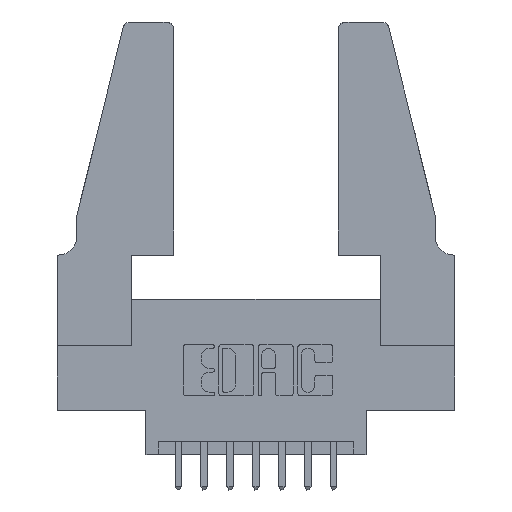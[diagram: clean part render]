
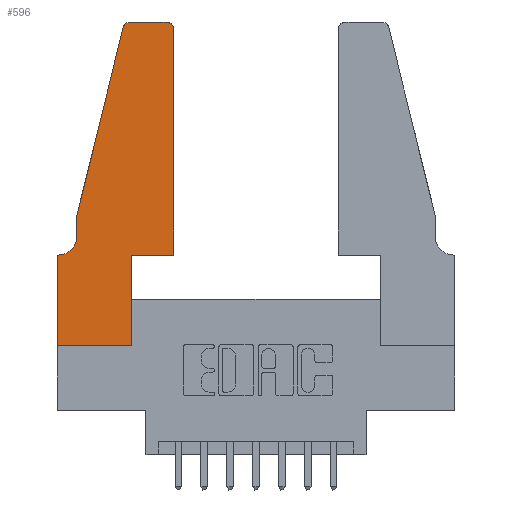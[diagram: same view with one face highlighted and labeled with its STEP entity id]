
A CAD part, top view. The second image highlights one B-rep face of the part: STEP entity #596.
In plain terms, the highlighted planar face has unit normal (0, 0, 1).
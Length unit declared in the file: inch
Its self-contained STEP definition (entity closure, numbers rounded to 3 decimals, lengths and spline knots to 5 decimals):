
#3 = LINE ( 'NONE', #2616, #12503 ) ;
#72 = VECTOR ( 'NONE', #836, 39.37008 ) ;
#285 = VERTEX_POINT ( 'NONE', #7904 ) ;
#545 = CARTESIAN_POINT ( 'NONE',  ( 0., 0., 0.37 ) ) ;
#596 = ADVANCED_FACE ( 'NONE', ( #7240 ), #2497, .T. ) ;
#632 = CIRCLE ( 'NONE', #2357, 0.07 ) ;
#703 = DIRECTION ( 'NONE',  ( 0., -1., 0. ) ) ;
#830 = DIRECTION ( 'NONE',  ( -1., 0., 0. ) ) ;
#836 = DIRECTION ( 'NONE',  ( 1., 0., 0. ) ) ;
#1062 = CARTESIAN_POINT ( 'NONE',  ( 0.0755, 0.42, 0.37 ) ) ;
#1194 = ORIENTED_EDGE ( 'NONE', *, *, #9621, .T. ) ;
#1334 = CARTESIAN_POINT ( 'NONE',  ( 0.4505, 0.35, 0.37 ) ) ;
#1351 = DIRECTION ( 'NONE',  ( 0., 1., 0. ) ) ;
#1478 = CARTESIAN_POINT ( 'NONE',  ( 0.4505, 0.35, 0.37 ) ) ;
#1559 = CARTESIAN_POINT ( 'NONE',  ( 0.4505, 1.22, 0.37 ) ) ;
#1688 = ORIENTED_EDGE ( 'NONE', *, *, #3262, .T. ) ;
#1807 = EDGE_CURVE ( 'NONE', #3341, #2200, #9001, .T. ) ;
#1856 = ORIENTED_EDGE ( 'NONE', *, *, #2678, .T. ) ;
#2013 = EDGE_CURVE ( 'NONE', #2795, #11368, #11263, .T. ) ;
#2200 = VERTEX_POINT ( 'NONE', #1062 ) ;
#2223 = VERTEX_POINT ( 'NONE', #3822 ) ;
#2312 = EDGE_CURVE ( 'NONE', #5438, #7473, #8326, .T. ) ;
#2357 = AXIS2_PLACEMENT_3D ( 'NONE', #5072, #4078, #9927 ) ;
#2497 = PLANE ( 'NONE',  #7299 ) ;
#2530 = CARTESIAN_POINT ( 'NONE',  ( 0.284, 1.22, 0.37 ) ) ;
#2616 = CARTESIAN_POINT ( 'NONE',  ( 0., 0., 0.37 ) ) ;
#2678 = EDGE_CURVE ( 'NONE', #2200, #5438, #632, .T. ) ;
#2680 = VECTOR ( 'NONE', #4739, 39.37008 ) ;
#2780 = ORIENTED_EDGE ( 'NONE', *, *, #2312, .T. ) ;
#2795 = VERTEX_POINT ( 'NONE', #545 ) ;
#3213 = EDGE_CURVE ( 'NONE', #6427, #285, #8364, .T. ) ;
#3262 = EDGE_CURVE ( 'NONE', #12402, #2223, #9408, .T. ) ;
#3292 = ORIENTED_EDGE ( 'NONE', *, *, #2013, .T. ) ;
#3341 = VERTEX_POINT ( 'NONE', #4653 ) ;
#3409 = CARTESIAN_POINT ( 'NONE',  ( 0.2865, 0., 0.37 ) ) ;
#3668 = EDGE_CURVE ( 'NONE', #7473, #2795, #3, .T. ) ;
#3670 = CARTESIAN_POINT ( 'NONE',  ( 0.284, 1.25, 0.37 ) ) ;
#3787 = EDGE_CURVE ( 'NONE', #5782, #5956, #7273, .T. ) ;
#3812 = LINE ( 'NONE', #5232, #6368 ) ;
#3822 = CARTESIAN_POINT ( 'NONE',  ( 0.25487, 1.22718, 0.37 ) ) ;
#3830 = VECTOR ( 'NONE', #9190, 39.37008 ) ;
#3849 = ORIENTED_EDGE ( 'NONE', *, *, #3213, .T. ) ;
#4078 = DIRECTION ( 'NONE',  ( 0., 0., -1. ) ) ;
#4103 = ORIENTED_EDGE ( 'NONE', *, *, #3787, .T. ) ;
#4184 = AXIS2_PLACEMENT_3D ( 'NONE', #5193, #6030, #5018 ) ;
#4193 = DIRECTION ( 'NONE',  ( -0.239, -0.971, 0. ) ) ;
#4235 = ORIENTED_EDGE ( 'NONE', *, *, #3668, .T. ) ;
#4653 = CARTESIAN_POINT ( 'NONE',  ( 0.0755, 0.5, 0.37 ) ) ;
#4739 = DIRECTION ( 'NONE',  ( 0., -1., 0. ) ) ;
#4747 = DIRECTION ( 'NONE',  ( 1., 0., 0. ) ) ;
#5018 = DIRECTION ( 'NONE',  ( 1., 0., 0. ) ) ;
#5052 = EDGE_CURVE ( 'NONE', #285, #5782, #9094, .T. ) ;
#5072 = CARTESIAN_POINT ( 'NONE',  ( 0.0055, 0.42, 0.37 ) ) ;
#5157 = VECTOR ( 'NONE', #1351, 39.37008 ) ;
#5193 = CARTESIAN_POINT ( 'NONE',  ( 0.4205, 1.22, 0.37 ) ) ;
#5232 = CARTESIAN_POINT ( 'NONE',  ( 0.0755, 0.5, 0.37 ) ) ;
#5438 = VERTEX_POINT ( 'NONE', #10940 ) ;
#5498 = EDGE_CURVE ( 'NONE', #11368, #6427, #9887, .T. ) ;
#5762 = VECTOR ( 'NONE', #830, 39.37008 ) ;
#5782 = VERTEX_POINT ( 'NONE', #1559 ) ;
#5956 = VERTEX_POINT ( 'NONE', #6002 ) ;
#5998 = ORIENTED_EDGE ( 'NONE', *, *, #5498, .T. ) ;
#6002 = CARTESIAN_POINT ( 'NONE',  ( 0.4205, 1.25, 0.37 ) ) ;
#6028 = ORIENTED_EDGE ( 'NONE', *, *, #11855, .T. ) ;
#6030 = DIRECTION ( 'NONE',  ( 0., 0., 1. ) ) ;
#6228 = VECTOR ( 'NONE', #9067, 39.37008 ) ;
#6342 = DIRECTION ( 'NONE',  ( 0., 0., 1. ) ) ;
#6368 = VECTOR ( 'NONE', #4193, 39.37008 ) ;
#6405 = VECTOR ( 'NONE', #10392, 39.37008 ) ;
#6427 = VERTEX_POINT ( 'NONE', #8842 ) ;
#6461 = CARTESIAN_POINT ( 'NONE',  ( 0., 0.35, 0.37 ) ) ;
#6505 = CARTESIAN_POINT ( 'NONE',  ( 0., 0., 0.37 ) ) ;
#7240 = FACE_OUTER_BOUND ( 'NONE', #7708, .T. ) ;
#7273 = CIRCLE ( 'NONE', #4184, 0.03 ) ;
#7289 = ORIENTED_EDGE ( 'NONE', *, *, #5052, .T. ) ;
#7299 = AXIS2_PLACEMENT_3D ( 'NONE', #6461, #6342, #4747 ) ;
#7317 = CARTESIAN_POINT ( 'NONE',  ( 0.2605, 1.25, 0.37 ) ) ;
#7473 = VERTEX_POINT ( 'NONE', #9739 ) ;
#7585 = CARTESIAN_POINT ( 'NONE',  ( 0.0755, 0.35, 0.37 ) ) ;
#7708 = EDGE_LOOP ( 'NONE', ( #1194, #1688, #6028, #8009, #1856, #2780, #4235, #3292, #5998, #3849, #7289, #4103 ) ) ;
#7882 = CARTESIAN_POINT ( 'NONE',  ( 0.2865, 0.35, 0.37 ) ) ;
#7904 = CARTESIAN_POINT ( 'NONE',  ( 0.4505, 0.35, 0.37 ) ) ;
#8009 = ORIENTED_EDGE ( 'NONE', *, *, #1807, .T. ) ;
#8326 = LINE ( 'NONE', #7585, #5762 ) ;
#8364 = LINE ( 'NONE', #1334, #6228 ) ;
#8842 = CARTESIAN_POINT ( 'NONE',  ( 0.2865, 0.35, 0.37 ) ) ;
#9001 = LINE ( 'NONE', #10667, #2680 ) ;
#9067 = DIRECTION ( 'NONE',  ( 1., 0., 0. ) ) ;
#9094 = LINE ( 'NONE', #1478, #5157 ) ;
#9190 = DIRECTION ( 'NONE',  ( 0., 1., 0. ) ) ;
#9408 = CIRCLE ( 'NONE', #11858, 0.03 ) ;
#9447 = DIRECTION ( 'NONE',  ( 1., 0., 0. ) ) ;
#9621 = EDGE_CURVE ( 'NONE', #5956, #12402, #9750, .T. ) ;
#9739 = CARTESIAN_POINT ( 'NONE',  ( 0., 0.35, 0.37 ) ) ;
#9750 = LINE ( 'NONE', #7317, #6405 ) ;
#9887 = LINE ( 'NONE', #7882, #3830 ) ;
#9927 = DIRECTION ( 'NONE',  ( -1., 0., 0. ) ) ;
#10392 = DIRECTION ( 'NONE',  ( -1., 0., 0. ) ) ;
#10667 = CARTESIAN_POINT ( 'NONE',  ( 0.0755, 0.5, 0.37 ) ) ;
#10940 = CARTESIAN_POINT ( 'NONE',  ( 0.0055, 0.35, 0.37 ) ) ;
#11263 = LINE ( 'NONE', #6505, #72 ) ;
#11290 = DIRECTION ( 'NONE',  ( 0., 0., 1. ) ) ;
#11368 = VERTEX_POINT ( 'NONE', #3409 ) ;
#11855 = EDGE_CURVE ( 'NONE', #2223, #3341, #3812, .T. ) ;
#11858 = AXIS2_PLACEMENT_3D ( 'NONE', #2530, #11290, #9447 ) ;
#12402 = VERTEX_POINT ( 'NONE', #3670 ) ;
#12503 = VECTOR ( 'NONE', #703, 39.37008 ) ;
